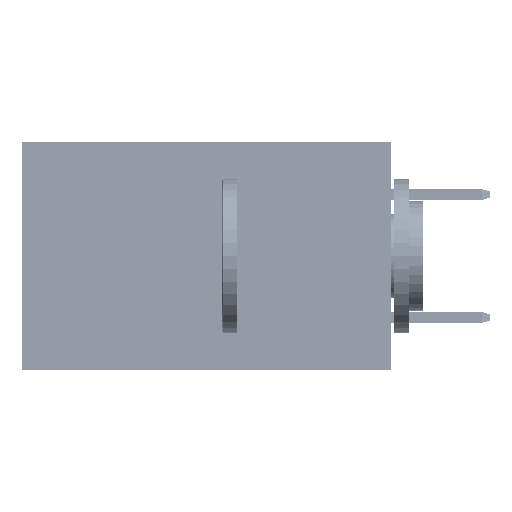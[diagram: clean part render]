
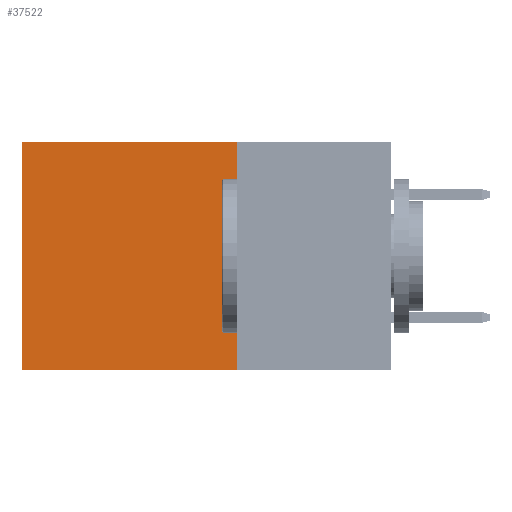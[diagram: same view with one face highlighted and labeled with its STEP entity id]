
A CAD part, left-side view. The second image highlights one B-rep face of the part: STEP entity #37522.
In plain terms, the highlighted planar face has unit normal (-1, 0, 0).
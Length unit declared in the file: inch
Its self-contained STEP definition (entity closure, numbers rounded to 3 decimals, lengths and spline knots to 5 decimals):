
#1106 = DIRECTION ( 'NONE',  ( 0., 0., -1. ) ) ;
#1912 = DIRECTION ( 'NONE',  ( 0., 0., -1. ) ) ;
#2008 = ORIENTED_EDGE ( 'NONE', *, *, #5586, .T. ) ;
#3686 = VECTOR ( 'NONE', #21784, 39.37008 ) ;
#5586 = EDGE_CURVE ( 'NONE', #44190, #7457, #31973, .T. ) ;
#6534 = CARTESIAN_POINT ( 'NONE',  ( 0.2875, 0.6, 0. ) ) ;
#6877 = LINE ( 'NONE', #16971, #8096 ) ;
#7457 = VERTEX_POINT ( 'NONE', #6534 ) ;
#8096 = VECTOR ( 'NONE', #1912, 39.37008 ) ;
#8457 = VECTOR ( 'NONE', #13220, 39.37008 ) ;
#9194 = CARTESIAN_POINT ( 'NONE',  ( 0.2875, 0.25, 0. ) ) ;
#10807 = VERTEX_POINT ( 'NONE', #41768 ) ;
#12263 = EDGE_CURVE ( 'NONE', #7457, #28583, #6877, .T. ) ;
#13220 = DIRECTION ( 'NONE',  ( 0., 1., 0. ) ) ;
#14262 = ORIENTED_EDGE ( 'NONE', *, *, #12263, .T. ) ;
#16971 = CARTESIAN_POINT ( 'NONE',  ( 0.2875, 0.6, 0. ) ) ;
#18970 = EDGE_CURVE ( 'NONE', #44190, #10807, #30912, .T. ) ;
#21784 = DIRECTION ( 'NONE',  ( 0., 0., -1. ) ) ;
#23284 = CARTESIAN_POINT ( 'NONE',  ( 0.2875, 0.25, 0. ) ) ;
#25654 = CARTESIAN_POINT ( 'NONE',  ( 0.2875, 0.25, 0. ) ) ;
#28583 = VERTEX_POINT ( 'NONE', #47175 ) ;
#28877 = EDGE_CURVE ( 'NONE', #10807, #28583, #43681, .T. ) ;
#29282 = CARTESIAN_POINT ( 'NONE',  ( 0.2875, 0.25, 0. ) ) ;
#30912 = LINE ( 'NONE', #25654, #3686 ) ;
#31973 = LINE ( 'NONE', #29282, #8457 ) ;
#32219 = VECTOR ( 'NONE', #41879, 39.37008 ) ;
#32671 = PLANE ( 'NONE',  #33674 ) ;
#33095 = EDGE_LOOP ( 'NONE', ( #14262, #41355, #48555, #2008 ) ) ;
#33674 = AXIS2_PLACEMENT_3D ( 'NONE', #9194, #43802, #1106 ) ;
#37522 = ADVANCED_FACE ( 'NONE', ( #47002 ), #32671, .F. ) ;
#38162 = CARTESIAN_POINT ( 'NONE',  ( 0.2875, 0.25, -0.37 ) ) ;
#41355 = ORIENTED_EDGE ( 'NONE', *, *, #28877, .F. ) ;
#41768 = CARTESIAN_POINT ( 'NONE',  ( 0.2875, 0.25, -0.37 ) ) ;
#41879 = DIRECTION ( 'NONE',  ( 0., 1., 0. ) ) ;
#43681 = LINE ( 'NONE', #38162, #32219 ) ;
#43802 = DIRECTION ( 'NONE',  ( 1., 0., 0. ) ) ;
#44190 = VERTEX_POINT ( 'NONE', #23284 ) ;
#47002 = FACE_OUTER_BOUND ( 'NONE', #33095, .T. ) ;
#47175 = CARTESIAN_POINT ( 'NONE',  ( 0.2875, 0.6, -0.37 ) ) ;
#48555 = ORIENTED_EDGE ( 'NONE', *, *, #18970, .F. ) ;
